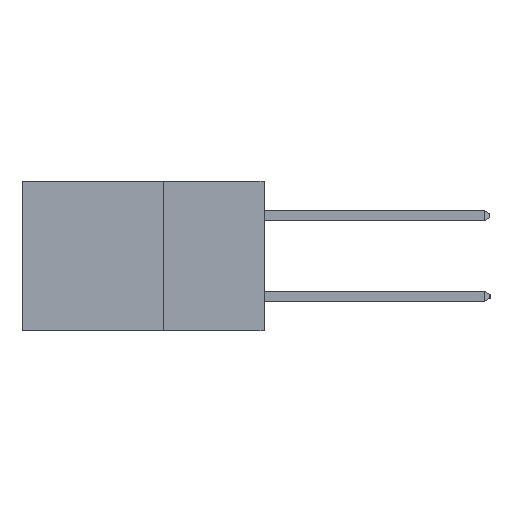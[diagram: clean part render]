
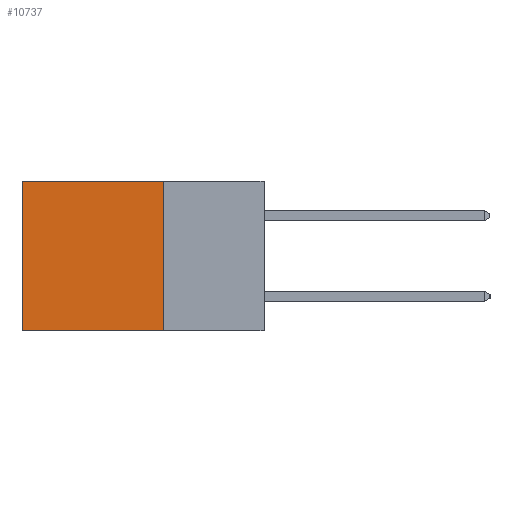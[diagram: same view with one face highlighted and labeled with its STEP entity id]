
A CAD part, left-side view. The second image highlights one B-rep face of the part: STEP entity #10737.
In plain terms, the highlighted planar face has unit normal (-1, 0, 0).
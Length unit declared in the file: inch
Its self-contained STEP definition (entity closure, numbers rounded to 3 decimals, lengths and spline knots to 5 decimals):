
#212 = CARTESIAN_POINT ( 'NONE',  ( 0.2615, 0.25, 0. ) ) ;
#318 = VERTEX_POINT ( 'NONE', #18510 ) ;
#1050 = LINE ( 'NONE', #18384, #6911 ) ;
#2069 = ORIENTED_EDGE ( 'NONE', *, *, #4873, .F. ) ;
#2201 = EDGE_CURVE ( 'NONE', #6977, #17435, #4271, .T. ) ;
#2459 = DIRECTION ( 'NONE',  ( 0., 0., -1. ) ) ;
#3871 = AXIS2_PLACEMENT_3D ( 'NONE', #10475, #12129, #2459 ) ;
#4024 = CARTESIAN_POINT ( 'NONE',  ( 0.2615, 0.6, -0.37 ) ) ;
#4271 = LINE ( 'NONE', #15784, #11830 ) ;
#4873 = EDGE_CURVE ( 'NONE', #6977, #8186, #19762, .T. ) ;
#5127 = DIRECTION ( 'NONE',  ( 0., 1., 0. ) ) ;
#6911 = VECTOR ( 'NONE', #10237, 39.37008 ) ;
#6977 = VERTEX_POINT ( 'NONE', #212 ) ;
#7012 = VECTOR ( 'NONE', #7265, 39.37008 ) ;
#7265 = DIRECTION ( 'NONE',  ( 0., 0., -1. ) ) ;
#8186 = VERTEX_POINT ( 'NONE', #17921 ) ;
#8220 = ORIENTED_EDGE ( 'NONE', *, *, #19232, .F. ) ;
#8853 = PLANE ( 'NONE',  #3871 ) ;
#10131 = ORIENTED_EDGE ( 'NONE', *, *, #12685, .T. ) ;
#10237 = DIRECTION ( 'NONE',  ( 0., 1., 0. ) ) ;
#10475 = CARTESIAN_POINT ( 'NONE',  ( 0.2615, 0.25, -0.37 ) ) ;
#10737 = ADVANCED_FACE ( 'NONE', ( #18195 ), #8853, .F. ) ;
#11830 = VECTOR ( 'NONE', #5127, 39.37008 ) ;
#12129 = DIRECTION ( 'NONE',  ( 1., 0., 0. ) ) ;
#12559 = DIRECTION ( 'NONE',  ( 0., 0., -1. ) ) ;
#12685 = EDGE_CURVE ( 'NONE', #17435, #318, #15621, .T. ) ;
#12706 = EDGE_LOOP ( 'NONE', ( #10131, #8220, #2069, #18777 ) ) ;
#12795 = CARTESIAN_POINT ( 'NONE',  ( 0.2615, 0.25, -0.37 ) ) ;
#15621 = LINE ( 'NONE', #4024, #7012 ) ;
#15784 = CARTESIAN_POINT ( 'NONE',  ( 0.2615, 0.25, 0. ) ) ;
#16048 = VECTOR ( 'NONE', #12559, 39.37008 ) ;
#17435 = VERTEX_POINT ( 'NONE', #20309 ) ;
#17921 = CARTESIAN_POINT ( 'NONE',  ( 0.2615, 0.25, -0.37 ) ) ;
#18195 = FACE_OUTER_BOUND ( 'NONE', #12706, .T. ) ;
#18384 = CARTESIAN_POINT ( 'NONE',  ( 0.2615, 0.25, -0.37 ) ) ;
#18510 = CARTESIAN_POINT ( 'NONE',  ( 0.2615, 0.6, -0.37 ) ) ;
#18777 = ORIENTED_EDGE ( 'NONE', *, *, #2201, .T. ) ;
#19232 = EDGE_CURVE ( 'NONE', #8186, #318, #1050, .T. ) ;
#19762 = LINE ( 'NONE', #12795, #16048 ) ;
#20309 = CARTESIAN_POINT ( 'NONE',  ( 0.2615, 0.6, 0. ) ) ;
